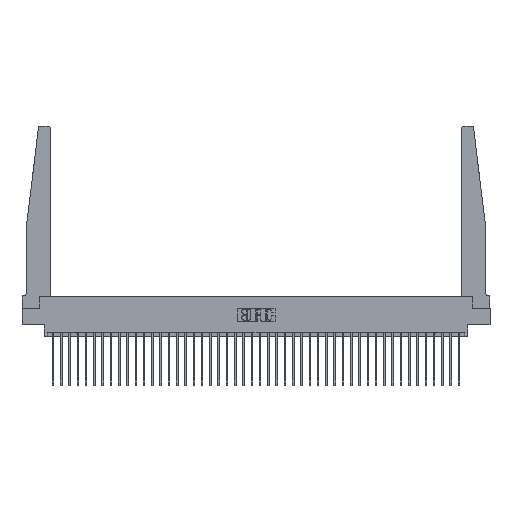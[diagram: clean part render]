
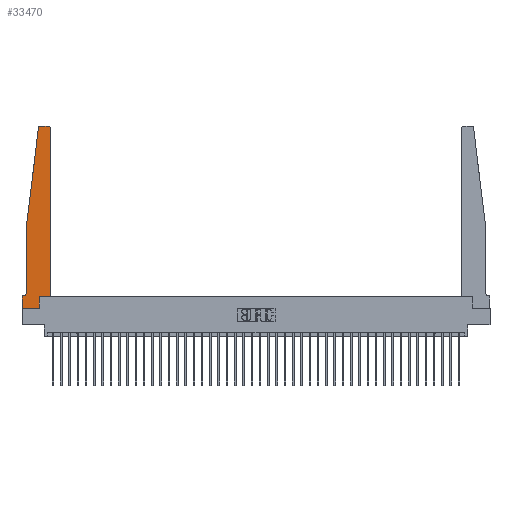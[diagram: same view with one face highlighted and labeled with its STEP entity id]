
A CAD part, top view. The second image highlights one B-rep face of the part: STEP entity #33470.
In plain terms, the highlighted planar face has unit normal (0, 0, 1).
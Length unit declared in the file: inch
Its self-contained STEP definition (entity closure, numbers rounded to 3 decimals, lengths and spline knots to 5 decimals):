
#34 = DIRECTION ( 'NONE',  ( 0., 0., 1. ) ) ;
#379 = LINE ( 'NONE', #15765, #29583 ) ;
#557 = LINE ( 'NONE', #14561, #8239 ) ;
#659 = LINE ( 'NONE', #26901, #22425 ) ;
#760 = CARTESIAN_POINT ( 'NONE',  ( 0.015, 0.1875, 0.37 ) ) ;
#1168 = FACE_OUTER_BOUND ( 'NONE', #19770, .T. ) ;
#1674 = EDGE_CURVE ( 'NONE', #11021, #3309, #659, .T. ) ;
#1816 = DIRECTION ( 'NONE',  ( 1., 0., 0. ) ) ;
#2322 = DIRECTION ( 'NONE',  ( 0., -1., 0. ) ) ;
#2902 = EDGE_CURVE ( 'NONE', #23627, #29949, #22779, .T. ) ;
#2985 = AXIS2_PLACEMENT_3D ( 'NONE', #12810, #32342, #15645 ) ;
#3309 = VERTEX_POINT ( 'NONE', #17034 ) ;
#3664 = CARTESIAN_POINT ( 'NONE',  ( 0.2605, 0.18, 0.37 ) ) ;
#3702 = CARTESIAN_POINT ( 'NONE',  ( 0.425, 0.18, 0.37 ) ) ;
#3749 = VERTEX_POINT ( 'NONE', #19553 ) ;
#3827 = CARTESIAN_POINT ( 'NONE',  ( 0.27653, 2.75, 0.37 ) ) ;
#3885 = EDGE_CURVE ( 'NONE', #17283, #3749, #557, .T. ) ;
#4634 = CARTESIAN_POINT ( 'NONE',  ( 0., 0.1875, 0.37 ) ) ;
#6499 = VERTEX_POINT ( 'NONE', #25951 ) ;
#6689 = DIRECTION ( 'NONE',  ( 0., 1., 0. ) ) ;
#7314 = AXIS2_PLACEMENT_3D ( 'NONE', #4634, #18861, #1816 ) ;
#8239 = VECTOR ( 'NONE', #28463, 39.37008 ) ;
#9734 = CARTESIAN_POINT ( 'NONE',  ( 0.065, 0.1875, 0.37 ) ) ;
#9752 = DIRECTION ( 'NONE',  ( 0., 0., -1. ) ) ;
#10808 = ORIENTED_EDGE ( 'NONE', *, *, #1674, .T. ) ;
#10862 = LINE ( 'NONE', #35959, #24909 ) ;
#10976 = VECTOR ( 'NONE', #12724, 39.37008 ) ;
#11021 = VERTEX_POINT ( 'NONE', #30738 ) ;
#11161 = CIRCLE ( 'NONE', #2985, 0.03 ) ;
#11537 = ORIENTED_EDGE ( 'NONE', *, *, #3885, .T. ) ;
#12348 = DIRECTION ( 'NONE',  ( -1., 0., 0. ) ) ;
#12390 = ORIENTED_EDGE ( 'NONE', *, *, #17399, .T. ) ;
#12724 = DIRECTION ( 'NONE',  ( -1., 0., 0. ) ) ;
#12810 = CARTESIAN_POINT ( 'NONE',  ( 0.27653, 2.72, 0.37 ) ) ;
#13091 = CARTESIAN_POINT ( 'NONE',  ( 0.24675, 2.72367, 0.37 ) ) ;
#13673 = EDGE_CURVE ( 'NONE', #15237, #17283, #35299, .T. ) ;
#13850 = CARTESIAN_POINT ( 'NONE',  ( 0.395, 2.75, 0.37 ) ) ;
#14175 = CIRCLE ( 'NONE', #23987, 0.03 ) ;
#14333 = LINE ( 'NONE', #3702, #35658 ) ;
#14561 = CARTESIAN_POINT ( 'NONE',  ( 0.425, 0.18, 0.37 ) ) ;
#15237 = VERTEX_POINT ( 'NONE', #30154 ) ;
#15645 = DIRECTION ( 'NONE',  ( 1., 0., 0. ) ) ;
#15765 = CARTESIAN_POINT ( 'NONE',  ( 0., 0., 0.37 ) ) ;
#16516 = ORIENTED_EDGE ( 'NONE', *, *, #29973, .T. ) ;
#17034 = CARTESIAN_POINT ( 'NONE',  ( 0., 0., 0.37 ) ) ;
#17153 = CARTESIAN_POINT ( 'NONE',  ( 0.395, 2.72, 0.37 ) ) ;
#17283 = VERTEX_POINT ( 'NONE', #36022 ) ;
#17293 = VERTEX_POINT ( 'NONE', #13850 ) ;
#17399 = EDGE_CURVE ( 'NONE', #6499, #17293, #14175, .T. ) ;
#17668 = VERTEX_POINT ( 'NONE', #3827 ) ;
#18463 = DIRECTION ( 'NONE',  ( 0., -1., 0. ) ) ;
#18464 = LINE ( 'NONE', #9734, #10976 ) ;
#18825 = LINE ( 'NONE', #26291, #29173 ) ;
#18861 = DIRECTION ( 'NONE',  ( 0., 0., 1. ) ) ;
#19553 = CARTESIAN_POINT ( 'NONE',  ( 0.425, 0.18, 0.37 ) ) ;
#19770 = EDGE_LOOP ( 'NONE', ( #23202, #22875, #26320, #33909, #23165, #28268, #10808, #20637, #29412, #11537, #16516, #12390 ) ) ;
#19945 = DIRECTION ( 'NONE',  ( 1., 0., 0. ) ) ;
#20637 = ORIENTED_EDGE ( 'NONE', *, *, #30178, .T. ) ;
#21411 = CARTESIAN_POINT ( 'NONE',  ( 0.065, 0.2375, 0.37 ) ) ;
#22078 = DIRECTION ( 'NONE',  ( -0.122, -0.992, 0. ) ) ;
#22127 = CARTESIAN_POINT ( 'NONE',  ( 0.065, 1.25, 0.37 ) ) ;
#22425 = VECTOR ( 'NONE', #18463, 39.37008 ) ;
#22779 = CIRCLE ( 'NONE', #25957, 0.05 ) ;
#22875 = ORIENTED_EDGE ( 'NONE', *, *, #32711, .T. ) ;
#23165 = ORIENTED_EDGE ( 'NONE', *, *, #2902, .T. ) ;
#23202 = ORIENTED_EDGE ( 'NONE', *, *, #29967, .T. ) ;
#23627 = VERTEX_POINT ( 'NONE', #21411 ) ;
#23987 = AXIS2_PLACEMENT_3D ( 'NONE', #17153, #34, #19945 ) ;
#24337 = VERTEX_POINT ( 'NONE', #22127 ) ;
#24909 = VECTOR ( 'NONE', #22078, 39.37008 ) ;
#24973 = CARTESIAN_POINT ( 'NONE',  ( 0.065, 1.25, 0.37 ) ) ;
#25847 = EDGE_CURVE ( 'NONE', #29508, #24337, #10862, .T. ) ;
#25951 = CARTESIAN_POINT ( 'NONE',  ( 0.425, 2.72, 0.37 ) ) ;
#25957 = AXIS2_PLACEMENT_3D ( 'NONE', #26575, #9752, #29383 ) ;
#26291 = CARTESIAN_POINT ( 'NONE',  ( 0.25, 2.75, 0.37 ) ) ;
#26320 = ORIENTED_EDGE ( 'NONE', *, *, #25847, .T. ) ;
#26575 = CARTESIAN_POINT ( 'NONE',  ( 0.015, 0.2375, 0.37 ) ) ;
#26901 = CARTESIAN_POINT ( 'NONE',  ( 0., 0., 0.37 ) ) ;
#27061 = PLANE ( 'NONE',  #7314 ) ;
#28268 = ORIENTED_EDGE ( 'NONE', *, *, #35042, .T. ) ;
#28463 = DIRECTION ( 'NONE',  ( 1., 0., 0. ) ) ;
#29094 = DIRECTION ( 'NONE',  ( 0., 1., 0. ) ) ;
#29173 = VECTOR ( 'NONE', #12348, 39.37008 ) ;
#29383 = DIRECTION ( 'NONE',  ( -1., 0., 0. ) ) ;
#29412 = ORIENTED_EDGE ( 'NONE', *, *, #13673, .T. ) ;
#29508 = VERTEX_POINT ( 'NONE', #13091 ) ;
#29583 = VECTOR ( 'NONE', #32466, 39.37008 ) ;
#29949 = VERTEX_POINT ( 'NONE', #760 ) ;
#29967 = EDGE_CURVE ( 'NONE', #17293, #17668, #18825, .T. ) ;
#29973 = EDGE_CURVE ( 'NONE', #3749, #6499, #14333, .T. ) ;
#30154 = CARTESIAN_POINT ( 'NONE',  ( 0.2605, 0., 0.37 ) ) ;
#30178 = EDGE_CURVE ( 'NONE', #3309, #15237, #379, .T. ) ;
#30738 = CARTESIAN_POINT ( 'NONE',  ( 0., 0.1875, 0.37 ) ) ;
#32342 = DIRECTION ( 'NONE',  ( 0., 0., 1. ) ) ;
#32466 = DIRECTION ( 'NONE',  ( 1., 0., 0. ) ) ;
#32711 = EDGE_CURVE ( 'NONE', #17668, #29508, #11161, .T. ) ;
#33470 = ADVANCED_FACE ( 'NONE', ( #1168 ), #27061, .T. ) ;
#33909 = ORIENTED_EDGE ( 'NONE', *, *, #34750, .T. ) ;
#34463 = VECTOR ( 'NONE', #6689, 39.37008 ) ;
#34640 = VECTOR ( 'NONE', #2322, 39.37008 ) ;
#34750 = EDGE_CURVE ( 'NONE', #24337, #23627, #35478, .T. ) ;
#35042 = EDGE_CURVE ( 'NONE', #29949, #11021, #18464, .T. ) ;
#35299 = LINE ( 'NONE', #3664, #34463 ) ;
#35478 = LINE ( 'NONE', #24973, #34640 ) ;
#35658 = VECTOR ( 'NONE', #29094, 39.37008 ) ;
#35959 = CARTESIAN_POINT ( 'NONE',  ( 0.065, 1.25, 0.37 ) ) ;
#36022 = CARTESIAN_POINT ( 'NONE',  ( 0.2605, 0.18, 0.37 ) ) ;
